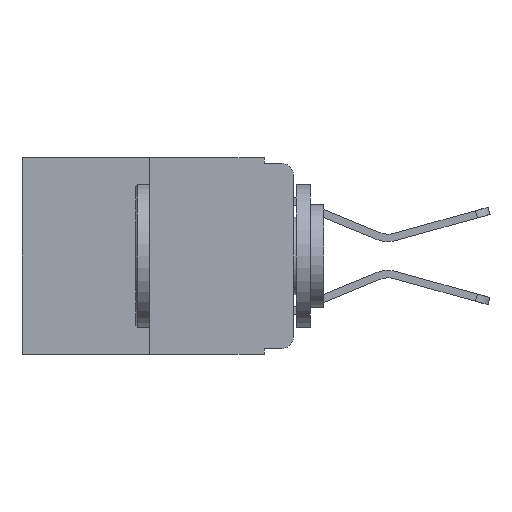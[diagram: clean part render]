
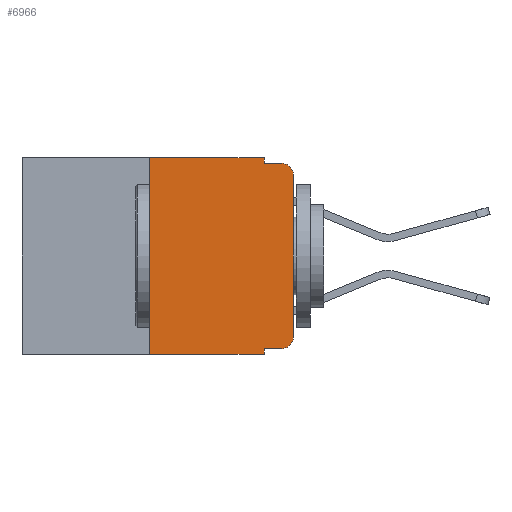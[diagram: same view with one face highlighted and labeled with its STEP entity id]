
A CAD part, left-side view. The second image highlights one B-rep face of the part: STEP entity #6966.
In plain terms, the highlighted planar face has unit normal (-1, 0, 0).
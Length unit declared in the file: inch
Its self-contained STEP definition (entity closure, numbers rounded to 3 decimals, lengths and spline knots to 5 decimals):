
#308 = CARTESIAN_POINT ( 'NONE',  ( 0., 0.25, 0. ) ) ;
#343 = EDGE_CURVE ( 'NONE', #505, #6935, #2343, .T. ) ;
#391 = EDGE_CURVE ( 'NONE', #6935, #5656, #7086, .T. ) ;
#415 = EDGE_CURVE ( 'NONE', #8843, #5656, #6472, .T. ) ;
#420 = EDGE_CURVE ( 'NONE', #3325, #8843, #11573, .T. ) ;
#441 = EDGE_CURVE ( 'NONE', #5284, #9492, #9087, .T. ) ;
#443 = EDGE_CURVE ( 'NONE', #10072, #995, #727, .T. ) ;
#456 = EDGE_CURVE ( 'NONE', #10072, #3027, #5830, .T. ) ;
#461 = EDGE_CURVE ( 'NONE', #3027, #505, #10997, .T. ) ;
#471 = DIRECTION ( 'NONE',  ( -1., 0., 0. ) ) ;
#505 = VERTEX_POINT ( 'NONE', #9789 ) ;
#727 = LINE ( 'NONE', #11181, #8458 ) ;
#869 = CARTESIAN_POINT ( 'NONE',  ( 0., 0.473, 0. ) ) ;
#995 = VERTEX_POINT ( 'NONE', #12234 ) ;
#1067 = VECTOR ( 'NONE', #12341, 39.37008 ) ;
#1094 = ORIENTED_EDGE ( 'NONE', *, *, #4368, .T. ) ;
#1172 = CARTESIAN_POINT ( 'NONE',  ( 0., 0.02, -0.03 ) ) ;
#1325 = CARTESIAN_POINT ( 'NONE',  ( 0., 0.02, -0.313 ) ) ;
#1354 = LINE ( 'NONE', #9078, #11543 ) ;
#1382 = CARTESIAN_POINT ( 'NONE',  ( 0., 0.051, -0.01 ) ) ;
#1385 = VECTOR ( 'NONE', #11167, 39.37008 ) ;
#1416 = AXIS2_PLACEMENT_3D ( 'NONE', #1325, #471, #3219 ) ;
#1497 = DIRECTION ( 'NONE',  ( -1., 0., 0. ) ) ;
#1514 = DIRECTION ( 'NONE',  ( 0., 0., -1. ) ) ;
#1738 = ORIENTED_EDGE ( 'NONE', *, *, #461, .T. ) ;
#1926 = DIRECTION ( 'NONE',  ( 0., 0., -1. ) ) ;
#2037 = VECTOR ( 'NONE', #9877, 39.37008 ) ;
#2041 = CARTESIAN_POINT ( 'NONE',  ( 0., 0.02, -0.01 ) ) ;
#2343 = LINE ( 'NONE', #7187, #2037 ) ;
#2518 = ORIENTED_EDGE ( 'NONE', *, *, #391, .T. ) ;
#2591 = EDGE_LOOP ( 'NONE', ( #12342, #2518, #7881, #10412, #2853, #6184, #1094, #3839, #11597, #1738 ) ) ;
#2609 = LINE ( 'NONE', #2957, #12699 ) ;
#2853 = ORIENTED_EDGE ( 'NONE', *, *, #3808, .F. ) ;
#2957 = CARTESIAN_POINT ( 'NONE',  ( 0., 0.473, -0.343 ) ) ;
#3027 = VERTEX_POINT ( 'NONE', #3887 ) ;
#3219 = DIRECTION ( 'NONE',  ( 0., 0., -1. ) ) ;
#3325 = VERTEX_POINT ( 'NONE', #8147 ) ;
#3514 = CARTESIAN_POINT ( 'NONE',  ( 0., 0.25, -0.343 ) ) ;
#3808 = EDGE_CURVE ( 'NONE', #9492, #3325, #1354, .T. ) ;
#3839 = ORIENTED_EDGE ( 'NONE', *, *, #443, .F. ) ;
#3887 = CARTESIAN_POINT ( 'NONE',  ( 0., 0.02, -0.333 ) ) ;
#4245 = FACE_OUTER_BOUND ( 'NONE', #2591, .T. ) ;
#4368 = EDGE_CURVE ( 'NONE', #5284, #995, #2609, .T. ) ;
#4906 = CARTESIAN_POINT ( 'NONE',  ( 0., 0., -0.03 ) ) ;
#5284 = VERTEX_POINT ( 'NONE', #3514 ) ;
#5656 = VERTEX_POINT ( 'NONE', #2041 ) ;
#5830 = LINE ( 'NONE', #8894, #11284 ) ;
#5944 = PLANE ( 'NONE',  #6525 ) ;
#6184 = ORIENTED_EDGE ( 'NONE', *, *, #441, .F. ) ;
#6472 = LINE ( 'NONE', #9270, #1385 ) ;
#6525 = AXIS2_PLACEMENT_3D ( 'NONE', #869, #7947, #1926 ) ;
#6935 = VERTEX_POINT ( 'NONE', #4906 ) ;
#6966 = ADVANCED_FACE ( 'NONE', ( #4245 ), #5944, .F. ) ;
#7086 = CIRCLE ( 'NONE', #9710, 0.02 ) ;
#7187 = CARTESIAN_POINT ( 'NONE',  ( 0., 0., 0. ) ) ;
#7450 = CARTESIAN_POINT ( 'NONE',  ( 0., 0.051, -0.333 ) ) ;
#7881 = ORIENTED_EDGE ( 'NONE', *, *, #415, .F. ) ;
#7947 = DIRECTION ( 'NONE',  ( 1., 0., 0. ) ) ;
#8147 = CARTESIAN_POINT ( 'NONE',  ( 0., 0.051, 0. ) ) ;
#8458 = VECTOR ( 'NONE', #10800, 39.37008 ) ;
#8769 = VECTOR ( 'NONE', #10765, 39.37008 ) ;
#8843 = VERTEX_POINT ( 'NONE', #1382 ) ;
#8894 = CARTESIAN_POINT ( 'NONE',  ( 0., 0.051, -0.333 ) ) ;
#9078 = CARTESIAN_POINT ( 'NONE',  ( 0., 0.473, 0. ) ) ;
#9087 = LINE ( 'NONE', #10787, #8769 ) ;
#9270 = CARTESIAN_POINT ( 'NONE',  ( 0., 0.051, -0.01 ) ) ;
#9444 = CARTESIAN_POINT ( 'NONE',  ( 0., 0.051, 0. ) ) ;
#9492 = VERTEX_POINT ( 'NONE', #308 ) ;
#9710 = AXIS2_PLACEMENT_3D ( 'NONE', #1172, #1497, #1514 ) ;
#9789 = CARTESIAN_POINT ( 'NONE',  ( 0., 0., -0.313 ) ) ;
#9877 = DIRECTION ( 'NONE',  ( 0., 0., 1. ) ) ;
#10072 = VERTEX_POINT ( 'NONE', #7450 ) ;
#10412 = ORIENTED_EDGE ( 'NONE', *, *, #420, .F. ) ;
#10765 = DIRECTION ( 'NONE',  ( 0., 0., 1. ) ) ;
#10787 = CARTESIAN_POINT ( 'NONE',  ( 0., 0.25, 0. ) ) ;
#10800 = DIRECTION ( 'NONE',  ( 0., 0., -1. ) ) ;
#10815 = DIRECTION ( 'NONE',  ( 0., -1., 0. ) ) ;
#10997 = CIRCLE ( 'NONE', #1416, 0.02 ) ;
#11167 = DIRECTION ( 'NONE',  ( 0., -1., 0. ) ) ;
#11181 = CARTESIAN_POINT ( 'NONE',  ( 0., 0.051, 0. ) ) ;
#11284 = VECTOR ( 'NONE', #10815, 39.37008 ) ;
#11543 = VECTOR ( 'NONE', #11575, 39.37008 ) ;
#11573 = LINE ( 'NONE', #9444, #1067 ) ;
#11575 = DIRECTION ( 'NONE',  ( 0., -1., 0. ) ) ;
#11597 = ORIENTED_EDGE ( 'NONE', *, *, #456, .T. ) ;
#11788 = DIRECTION ( 'NONE',  ( 0., -1., 0. ) ) ;
#12234 = CARTESIAN_POINT ( 'NONE',  ( 0., 0.051, -0.343 ) ) ;
#12341 = DIRECTION ( 'NONE',  ( 0., 0., -1. ) ) ;
#12342 = ORIENTED_EDGE ( 'NONE', *, *, #343, .T. ) ;
#12699 = VECTOR ( 'NONE', #11788, 39.37008 ) ;
